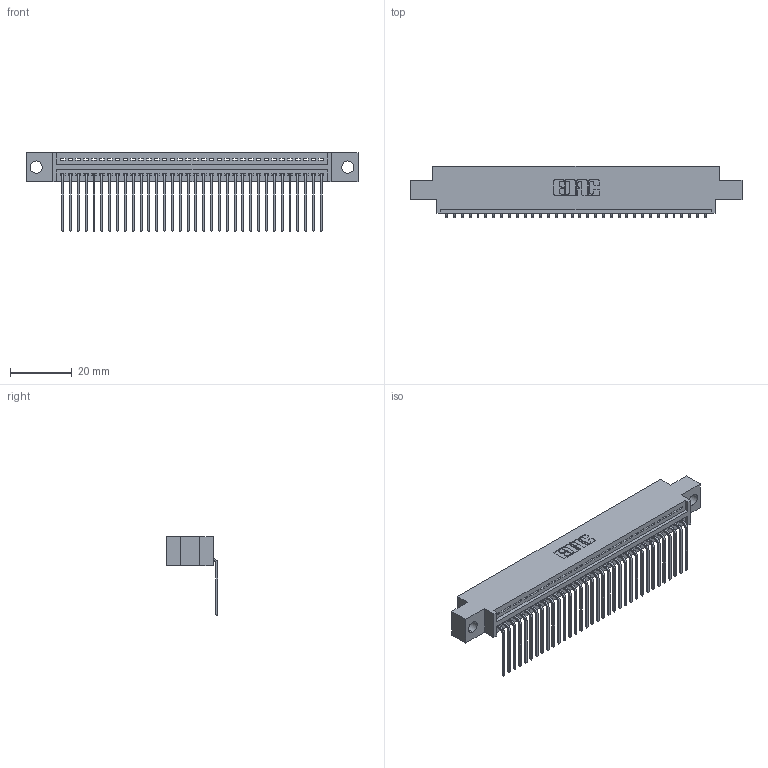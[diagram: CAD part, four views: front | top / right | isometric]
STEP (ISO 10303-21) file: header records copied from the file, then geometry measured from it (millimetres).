
FILE_DESCRIPTION (( 'STEP AP203' ), '1' );
FILE_NAME ('345-034-559-604.STEP', '2018-08-29T04:52:58', ( '' ), ( '' ), 'SwSTEP 2.0', 'SolidWorks 2016', '' );
FILE_SCHEMA (( 'CONFIG_CONTROL_DESIGN' ));
Length unit declared in the file: inch
Products named in the file (3): 345 Part_0.170 Offset - 0.156 Dia-TH; 345-292-001_558 559 Tail - 1; 345-034-559-604
Assembly tree (35 placements, depth 2):
  345-034-559-604
    345 Part_0.170 Offset - 0.156 Dia-TH
    345-292-001_558 559 Tail - 1  x34
Bounding box: 107.57 x 16.75 x 25.53 mm (x, y, z)
Volume: 10063.5 mm3; surface area: 13865.7 mm2
Topology: 35 solids, 35 shells, 2170 faces, 6541 edges, 4314 vertices
Faces by surface type: plane 1512, cylinder 658
Entity records: 26885 total; most frequent: CARTESIAN_POINT 4666, ORIENTED_EDGE 4634, DIRECTION 4085, EDGE_CURVE 2317, LINE 2049, VECTOR 2049, VERTEX_POINT 1542, AXIS2_PLACEMENT_3D 1018
